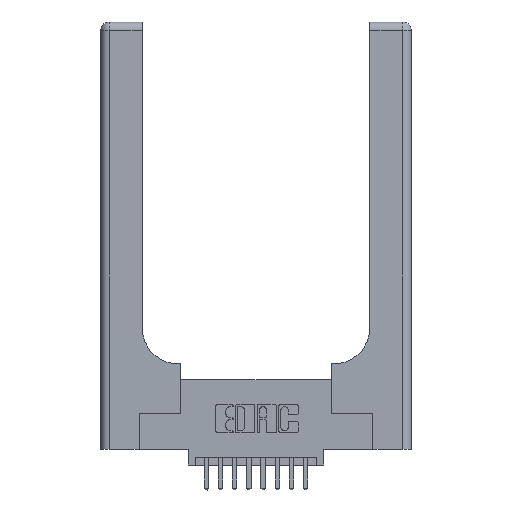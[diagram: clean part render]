
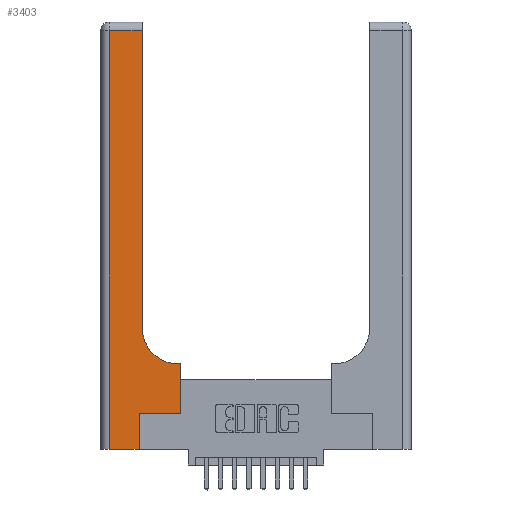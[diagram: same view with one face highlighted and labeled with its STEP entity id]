
A CAD part, top view. The second image highlights one B-rep face of the part: STEP entity #3403.
In plain terms, the highlighted planar face has unit normal (0, 0, 1).
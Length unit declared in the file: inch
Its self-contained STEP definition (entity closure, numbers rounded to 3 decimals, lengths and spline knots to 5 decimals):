
#220 = CARTESIAN_POINT ( 'NONE',  ( 0.269, 0., 0.37 ) ) ;
#322 = LINE ( 'NONE', #7720, #16261 ) ;
#416 = EDGE_CURVE ( 'NONE', #16214, #1422, #8441, .T. ) ;
#559 = ORIENTED_EDGE ( 'NONE', *, *, #15170, .T. ) ;
#1182 = DIRECTION ( 'NONE',  ( 1., 0., 0. ) ) ;
#1194 = ORIENTED_EDGE ( 'NONE', *, *, #6862, .T. ) ;
#1392 = DIRECTION ( 'NONE',  ( -1., 0., 0. ) ) ;
#1396 = LINE ( 'NONE', #4233, #4338 ) ;
#1422 = VERTEX_POINT ( 'NONE', #8464 ) ;
#1552 = ORIENTED_EDGE ( 'NONE', *, *, #9826, .T. ) ;
#1819 = VERTEX_POINT ( 'NONE', #9597 ) ;
#2014 = EDGE_CURVE ( 'NONE', #1422, #14199, #15233, .T. ) ;
#2166 = ORIENTED_EDGE ( 'NONE', *, *, #11849, .T. ) ;
#2264 = ORIENTED_EDGE ( 'NONE', *, *, #10941, .T. ) ;
#2612 = VERTEX_POINT ( 'NONE', #7345 ) ;
#2691 = LINE ( 'NONE', #10849, #9807 ) ;
#2706 = VERTEX_POINT ( 'NONE', #3736 ) ;
#2798 = ORIENTED_EDGE ( 'NONE', *, *, #416, .T. ) ;
#2918 = LINE ( 'NONE', #14869, #9232 ) ;
#2993 = LINE ( 'NONE', #220, #15610 ) ;
#3361 = FACE_OUTER_BOUND ( 'NONE', #8108, .T. ) ;
#3396 = CARTESIAN_POINT ( 'NONE',  ( 0., 3., 0.37 ) ) ;
#3403 = ADVANCED_FACE ( 'NONE', ( #3361 ), #10922, .F. ) ;
#3736 = CARTESIAN_POINT ( 'NONE',  ( 0.2915, 2.94, 0.37 ) ) ;
#4233 = CARTESIAN_POINT ( 'NONE',  ( 0., 2.94, 0.37 ) ) ;
#4338 = VECTOR ( 'NONE', #9315, 39.37008 ) ;
#4657 = DIRECTION ( 'NONE',  ( 0., 0., -1. ) ) ;
#5518 = CARTESIAN_POINT ( 'NONE',  ( 0.5585, 0.6, 0.37 ) ) ;
#5649 = LINE ( 'NONE', #8182, #11917 ) ;
#5727 = CARTESIAN_POINT ( 'NONE',  ( 0.2915, 3., 0.37 ) ) ;
#6029 = LINE ( 'NONE', #5727, #12287 ) ;
#6357 = ORIENTED_EDGE ( 'NONE', *, *, #14868, .T. ) ;
#6740 = CARTESIAN_POINT ( 'NONE',  ( 0.06, 2.94, 0.37 ) ) ;
#6862 = EDGE_CURVE ( 'NONE', #1819, #13328, #2691, .T. ) ;
#6996 = DIRECTION ( 'NONE',  ( 0., 1., 0. ) ) ;
#7344 = DIRECTION ( 'NONE',  ( 1., 0., 0. ) ) ;
#7345 = CARTESIAN_POINT ( 'NONE',  ( 0.06, 0., 0.37 ) ) ;
#7720 = CARTESIAN_POINT ( 'NONE',  ( 0.5585, 0.25, 0.37 ) ) ;
#8108 = EDGE_LOOP ( 'NONE', ( #559, #2264, #9265, #2166, #1552, #1194, #6357, #2798, #10857 ) ) ;
#8182 = CARTESIAN_POINT ( 'NONE',  ( 0.06, 3., 0.37 ) ) ;
#8441 = LINE ( 'NONE', #10195, #15124 ) ;
#8464 = CARTESIAN_POINT ( 'NONE',  ( 0.5415, 0.6, 0.37 ) ) ;
#8729 = DIRECTION ( 'NONE',  ( 0., 0., -1. ) ) ;
#8923 = AXIS2_PLACEMENT_3D ( 'NONE', #16260, #8729, #1182 ) ;
#8974 = DIRECTION ( 'NONE',  ( 0., 1., 0. ) ) ;
#9007 = DIRECTION ( 'NONE',  ( 0., 1., 0. ) ) ;
#9232 = VECTOR ( 'NONE', #7344, 39.37008 ) ;
#9256 = CARTESIAN_POINT ( 'NONE',  ( 0.269, 0., 0.37 ) ) ;
#9265 = ORIENTED_EDGE ( 'NONE', *, *, #14238, .T. ) ;
#9315 = DIRECTION ( 'NONE',  ( -1., 0., 0. ) ) ;
#9582 = DIRECTION ( 'NONE',  ( 1., 0., 0. ) ) ;
#9597 = CARTESIAN_POINT ( 'NONE',  ( 0.269, 0.25, 0.37 ) ) ;
#9807 = VECTOR ( 'NONE', #9582, 39.37008 ) ;
#9826 = EDGE_CURVE ( 'NONE', #16199, #1819, #2993, .T. ) ;
#10195 = CARTESIAN_POINT ( 'NONE',  ( 0.2915, 0.6, 0.37 ) ) ;
#10198 = AXIS2_PLACEMENT_3D ( 'NONE', #3396, #4657, #13466 ) ;
#10849 = CARTESIAN_POINT ( 'NONE',  ( 0.269, 0.25, 0.37 ) ) ;
#10857 = ORIENTED_EDGE ( 'NONE', *, *, #2014, .T. ) ;
#10922 = PLANE ( 'NONE',  #10198 ) ;
#10941 = EDGE_CURVE ( 'NONE', #2706, #11582, #1396, .T. ) ;
#11582 = VERTEX_POINT ( 'NONE', #6740 ) ;
#11670 = CARTESIAN_POINT ( 'NONE',  ( 0.5585, 0.25, 0.37 ) ) ;
#11849 = EDGE_CURVE ( 'NONE', #2612, #16199, #2918, .T. ) ;
#11917 = VECTOR ( 'NONE', #14497, 39.37008 ) ;
#12287 = VECTOR ( 'NONE', #6996, 39.37008 ) ;
#13328 = VERTEX_POINT ( 'NONE', #11670 ) ;
#13466 = DIRECTION ( 'NONE',  ( -1., 0., 0. ) ) ;
#14199 = VERTEX_POINT ( 'NONE', #14271 ) ;
#14238 = EDGE_CURVE ( 'NONE', #11582, #2612, #5649, .T. ) ;
#14271 = CARTESIAN_POINT ( 'NONE',  ( 0.2915, 0.85, 0.37 ) ) ;
#14497 = DIRECTION ( 'NONE',  ( 0., -1., 0. ) ) ;
#14868 = EDGE_CURVE ( 'NONE', #13328, #16214, #322, .T. ) ;
#14869 = CARTESIAN_POINT ( 'NONE',  ( 0., 0., 0.37 ) ) ;
#15124 = VECTOR ( 'NONE', #1392, 39.37008 ) ;
#15170 = EDGE_CURVE ( 'NONE', #14199, #2706, #6029, .T. ) ;
#15233 = CIRCLE ( 'NONE', #8923, 0.25 ) ;
#15610 = VECTOR ( 'NONE', #9007, 39.37008 ) ;
#16199 = VERTEX_POINT ( 'NONE', #9256 ) ;
#16214 = VERTEX_POINT ( 'NONE', #5518 ) ;
#16260 = CARTESIAN_POINT ( 'NONE',  ( 0.5415, 0.85, 0.37 ) ) ;
#16261 = VECTOR ( 'NONE', #8974, 39.37008 ) ;
